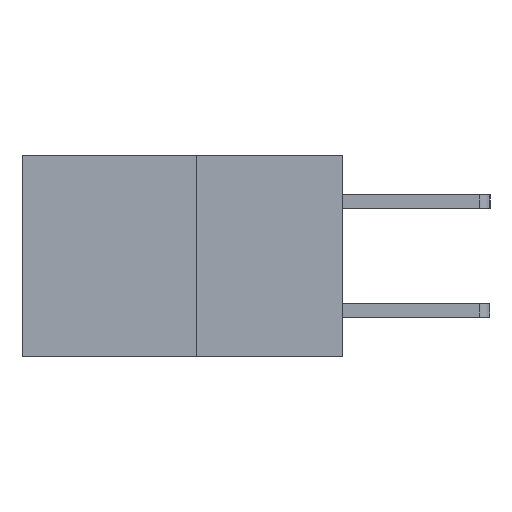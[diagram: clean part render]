
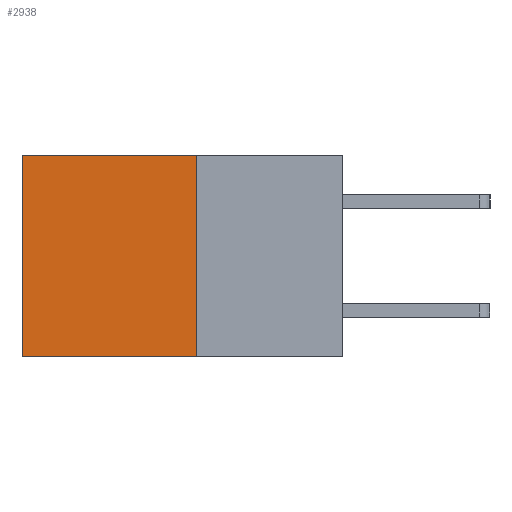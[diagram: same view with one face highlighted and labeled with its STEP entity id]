
A CAD part, left-side view. The second image highlights one B-rep face of the part: STEP entity #2938.
In plain terms, the highlighted planar face has unit normal (-1, 0, 0).
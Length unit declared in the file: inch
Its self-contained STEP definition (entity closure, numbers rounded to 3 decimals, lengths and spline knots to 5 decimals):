
#35 = EDGE_CURVE ( 'NONE', #6415, #3859, #7342, .T. ) ;
#252 = EDGE_CURVE ( 'NONE', #2807, #6415, #5206, .T. ) ;
#1411 = CARTESIAN_POINT ( 'NONE',  ( 0.277, 0.27, -0.37 ) ) ;
#1537 = ORIENTED_EDGE ( 'NONE', *, *, #3005, .F. ) ;
#1550 = EDGE_CURVE ( 'NONE', #2807, #2355, #7941, .T. ) ;
#2355 = VERTEX_POINT ( 'NONE', #8762 ) ;
#2807 = VERTEX_POINT ( 'NONE', #10212 ) ;
#2938 = ADVANCED_FACE ( 'NONE', ( #6928 ), #8640, .F. ) ;
#3005 = EDGE_CURVE ( 'NONE', #2355, #3859, #4081, .T. ) ;
#3842 = CARTESIAN_POINT ( 'NONE',  ( 0.277, 0.27, 0. ) ) ;
#3859 = VERTEX_POINT ( 'NONE', #7463 ) ;
#4031 = CARTESIAN_POINT ( 'NONE',  ( 0.277, 0.59, -0.37 ) ) ;
#4081 = LINE ( 'NONE', #7812, #11891 ) ;
#4173 = ORIENTED_EDGE ( 'NONE', *, *, #1550, .F. ) ;
#5206 = LINE ( 'NONE', #3842, #12003 ) ;
#5237 = VECTOR ( 'NONE', #6554, 39.37008 ) ;
#5386 = AXIS2_PLACEMENT_3D ( 'NONE', #9047, #8536, #8453 ) ;
#6415 = VERTEX_POINT ( 'NONE', #6622 ) ;
#6420 = DIRECTION ( 'NONE',  ( 0., 0., -1. ) ) ;
#6468 = ORIENTED_EDGE ( 'NONE', *, *, #35, .T. ) ;
#6554 = DIRECTION ( 'NONE',  ( 0., 0., -1. ) ) ;
#6622 = CARTESIAN_POINT ( 'NONE',  ( 0.277, 0.59, 0. ) ) ;
#6928 = FACE_OUTER_BOUND ( 'NONE', #8618, .T. ) ;
#7342 = LINE ( 'NONE', #4031, #12318 ) ;
#7463 = CARTESIAN_POINT ( 'NONE',  ( 0.277, 0.59, -0.37 ) ) ;
#7529 = DIRECTION ( 'NONE',  ( 0., 1., 0. ) ) ;
#7812 = CARTESIAN_POINT ( 'NONE',  ( 0.277, 0.27, -0.37 ) ) ;
#7941 = LINE ( 'NONE', #1411, #5237 ) ;
#8453 = DIRECTION ( 'NONE',  ( 0., 0., -1. ) ) ;
#8536 = DIRECTION ( 'NONE',  ( 1., 0., 0. ) ) ;
#8618 = EDGE_LOOP ( 'NONE', ( #6468, #1537, #4173, #9175 ) ) ;
#8640 = PLANE ( 'NONE',  #5386 ) ;
#8762 = CARTESIAN_POINT ( 'NONE',  ( 0.277, 0.27, -0.37 ) ) ;
#9047 = CARTESIAN_POINT ( 'NONE',  ( 0.277, 0.27, -0.37 ) ) ;
#9175 = ORIENTED_EDGE ( 'NONE', *, *, #252, .T. ) ;
#10146 = DIRECTION ( 'NONE',  ( 0., 1., 0. ) ) ;
#10212 = CARTESIAN_POINT ( 'NONE',  ( 0.277, 0.27, 0. ) ) ;
#11891 = VECTOR ( 'NONE', #7529, 39.37008 ) ;
#12003 = VECTOR ( 'NONE', #10146, 39.37008 ) ;
#12318 = VECTOR ( 'NONE', #6420, 39.37008 ) ;
